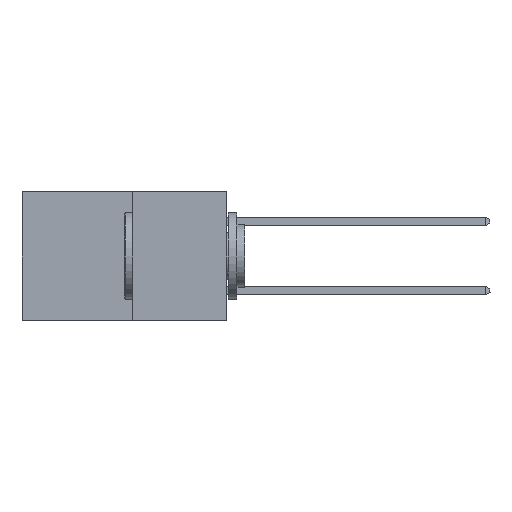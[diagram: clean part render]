
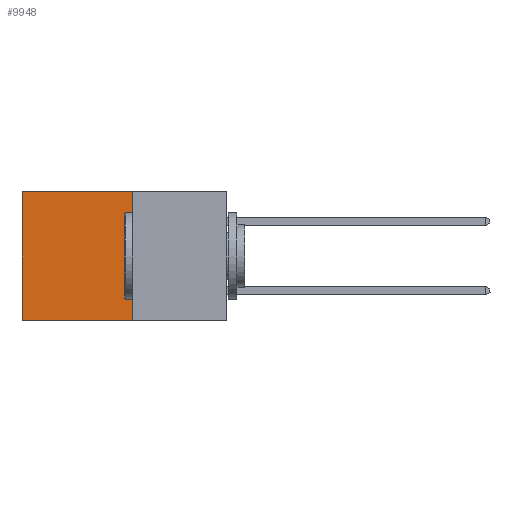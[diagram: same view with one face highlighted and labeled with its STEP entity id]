
A CAD part, left-side view. The second image highlights one B-rep face of the part: STEP entity #9948.
In plain terms, the highlighted planar face has unit normal (-1, 0, 0).
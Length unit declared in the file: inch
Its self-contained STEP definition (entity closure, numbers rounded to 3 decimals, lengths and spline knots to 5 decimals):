
#922 = EDGE_CURVE ( 'NONE', #8200, #14043, #10953, .T. ) ;
#2309 = LINE ( 'NONE', #25806, #20626 ) ;
#2406 = EDGE_LOOP ( 'NONE', ( #11733, #4565, #6799, #10653 ) ) ;
#3869 = CARTESIAN_POINT ( 'NONE',  ( 0.277, 0.59, -0.37 ) ) ;
#4029 = LINE ( 'NONE', #11051, #27781 ) ;
#4565 = ORIENTED_EDGE ( 'NONE', *, *, #15341, .F. ) ;
#6311 = DIRECTION ( 'NONE',  ( 0., 0., -1. ) ) ;
#6437 = VECTOR ( 'NONE', #6311, 39.37008 ) ;
#6799 = ORIENTED_EDGE ( 'NONE', *, *, #922, .F. ) ;
#7590 = PLANE ( 'NONE',  #20537 ) ;
#8200 = VERTEX_POINT ( 'NONE', #18740 ) ;
#8422 = VERTEX_POINT ( 'NONE', #14759 ) ;
#9948 = ADVANCED_FACE ( 'NONE', ( #27391 ), #7590, .F. ) ;
#9989 = DIRECTION ( 'NONE',  ( 0., 0., -1. ) ) ;
#10653 = ORIENTED_EDGE ( 'NONE', *, *, #22286, .T. ) ;
#10953 = LINE ( 'NONE', #21816, #16545 ) ;
#11051 = CARTESIAN_POINT ( 'NONE',  ( 0.277, 0.27, -0.37 ) ) ;
#11602 = DIRECTION ( 'NONE',  ( 0., 1., 0. ) ) ;
#11733 = ORIENTED_EDGE ( 'NONE', *, *, #21842, .T. ) ;
#12363 = VERTEX_POINT ( 'NONE', #25089 ) ;
#14043 = VERTEX_POINT ( 'NONE', #27726 ) ;
#14759 = CARTESIAN_POINT ( 'NONE',  ( 0.277, 0.59, 0. ) ) ;
#15341 = EDGE_CURVE ( 'NONE', #14043, #12363, #4029, .T. ) ;
#16545 = VECTOR ( 'NONE', #22325, 39.37008 ) ;
#18740 = CARTESIAN_POINT ( 'NONE',  ( 0.277, 0.27, 0. ) ) ;
#19122 = LINE ( 'NONE', #3869, #6437 ) ;
#19428 = CARTESIAN_POINT ( 'NONE',  ( 0.277, 0.27, -0.37 ) ) ;
#20537 = AXIS2_PLACEMENT_3D ( 'NONE', #19428, #24185, #9989 ) ;
#20626 = VECTOR ( 'NONE', #11602, 39.37008 ) ;
#21816 = CARTESIAN_POINT ( 'NONE',  ( 0.277, 0.27, -0.37 ) ) ;
#21842 = EDGE_CURVE ( 'NONE', #8422, #12363, #19122, .T. ) ;
#22286 = EDGE_CURVE ( 'NONE', #8200, #8422, #2309, .T. ) ;
#22325 = DIRECTION ( 'NONE',  ( 0., 0., -1. ) ) ;
#24185 = DIRECTION ( 'NONE',  ( 1., 0., 0. ) ) ;
#25089 = CARTESIAN_POINT ( 'NONE',  ( 0.277, 0.59, -0.37 ) ) ;
#25806 = CARTESIAN_POINT ( 'NONE',  ( 0.277, 0.27, 0. ) ) ;
#27391 = FACE_OUTER_BOUND ( 'NONE', #2406, .T. ) ;
#27726 = CARTESIAN_POINT ( 'NONE',  ( 0.277, 0.27, -0.37 ) ) ;
#27781 = VECTOR ( 'NONE', #29995, 39.37008 ) ;
#29995 = DIRECTION ( 'NONE',  ( 0., 1., 0. ) ) ;
